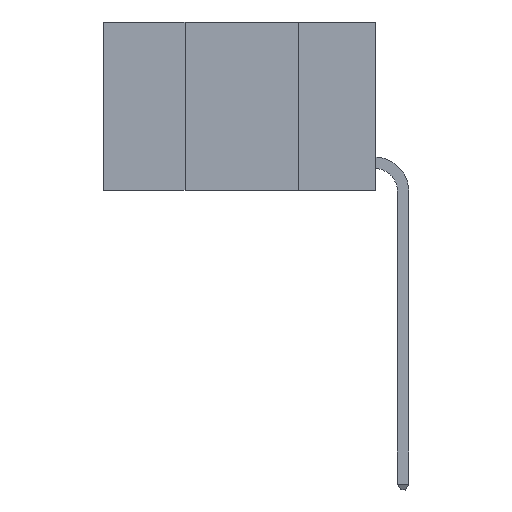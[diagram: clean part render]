
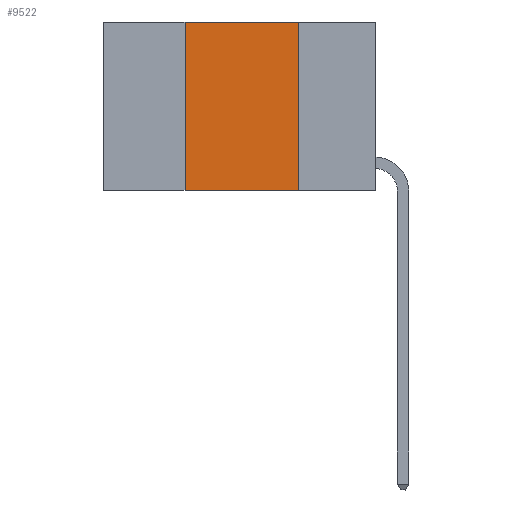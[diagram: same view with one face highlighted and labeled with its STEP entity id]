
A CAD part, left-side view. The second image highlights one B-rep face of the part: STEP entity #9522.
In plain terms, the highlighted planar face has unit normal (-1, 0, 0).
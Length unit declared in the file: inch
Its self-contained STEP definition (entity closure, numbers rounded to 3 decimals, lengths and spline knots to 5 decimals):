
#571 = PLANE ( 'NONE',  #10758 ) ;
#730 = CARTESIAN_POINT ( 'NONE',  ( 0., 0.42, 0. ) ) ;
#772 = CARTESIAN_POINT ( 'NONE',  ( 0., 0.17, 0. ) ) ;
#1085 = ORIENTED_EDGE ( 'NONE', *, *, #18060, .F. ) ;
#1265 = VERTEX_POINT ( 'NONE', #772 ) ;
#1496 = ORIENTED_EDGE ( 'NONE', *, *, #7381, .F. ) ;
#1718 = ORIENTED_EDGE ( 'NONE', *, *, #5365, .F. ) ;
#1789 = CARTESIAN_POINT ( 'NONE',  ( 0., 0.17, 0. ) ) ;
#1856 = CARTESIAN_POINT ( 'NONE',  ( 0., 0.6, -0.37 ) ) ;
#3310 = DIRECTION ( 'NONE',  ( 0., 0., -1. ) ) ;
#3374 = DIRECTION ( 'NONE',  ( 0., -1., 0. ) ) ;
#3626 = ORIENTED_EDGE ( 'NONE', *, *, #17790, .T. ) ;
#3776 = LINE ( 'NONE', #16267, #19224 ) ;
#5139 = LINE ( 'NONE', #1789, #16174 ) ;
#5365 = EDGE_CURVE ( 'NONE', #7028, #8897, #3776, .T. ) ;
#5432 = CARTESIAN_POINT ( 'NONE',  ( 0., 0.6, 0. ) ) ;
#5507 = FACE_OUTER_BOUND ( 'NONE', #19048, .T. ) ;
#6964 = CARTESIAN_POINT ( 'NONE',  ( 0., 0.42, -0.37 ) ) ;
#7028 = VERTEX_POINT ( 'NONE', #6964 ) ;
#7371 = CARTESIAN_POINT ( 'NONE',  ( 0., 0.17, -0.37 ) ) ;
#7381 = EDGE_CURVE ( 'NONE', #1265, #18858, #5139, .T. ) ;
#7543 = LINE ( 'NONE', #5432, #18064 ) ;
#7790 = LINE ( 'NONE', #1856, #18755 ) ;
#8189 = DIRECTION ( 'NONE',  ( 1., 0., 0. ) ) ;
#8785 = DIRECTION ( 'NONE',  ( 0., 0., 1. ) ) ;
#8897 = VERTEX_POINT ( 'NONE', #730 ) ;
#9522 = ADVANCED_FACE ( 'NONE', ( #5507 ), #571, .F. ) ;
#10758 = AXIS2_PLACEMENT_3D ( 'NONE', #17172, #8189, #18639 ) ;
#16174 = VECTOR ( 'NONE', #3310, 39.37008 ) ;
#16267 = CARTESIAN_POINT ( 'NONE',  ( 0., 0.42, 0. ) ) ;
#17172 = CARTESIAN_POINT ( 'NONE',  ( 0., 0.6, 0. ) ) ;
#17428 = DIRECTION ( 'NONE',  ( 0., -1., 0. ) ) ;
#17790 = EDGE_CURVE ( 'NONE', #7028, #18858, #7790, .T. ) ;
#18060 = EDGE_CURVE ( 'NONE', #8897, #1265, #7543, .T. ) ;
#18064 = VECTOR ( 'NONE', #17428, 39.37008 ) ;
#18639 = DIRECTION ( 'NONE',  ( 0., 0., -1. ) ) ;
#18755 = VECTOR ( 'NONE', #3374, 39.37008 ) ;
#18858 = VERTEX_POINT ( 'NONE', #7371 ) ;
#19048 = EDGE_LOOP ( 'NONE', ( #1496, #1085, #1718, #3626 ) ) ;
#19224 = VECTOR ( 'NONE', #8785, 39.37008 ) ;
